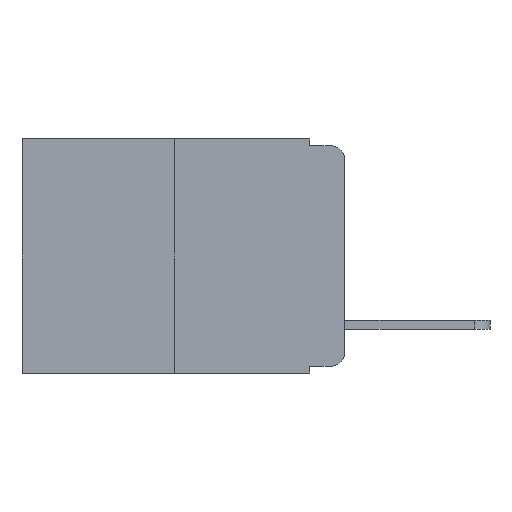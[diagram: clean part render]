
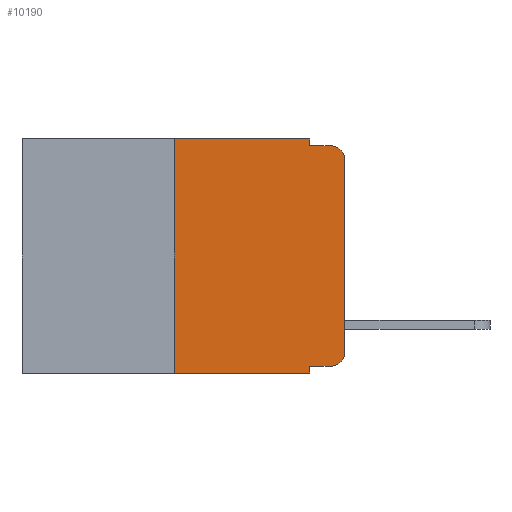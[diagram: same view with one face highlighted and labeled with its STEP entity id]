
A CAD part, left-side view. The second image highlights one B-rep face of the part: STEP entity #10190.
In plain terms, the highlighted planar face has unit normal (-1, 0, 0).
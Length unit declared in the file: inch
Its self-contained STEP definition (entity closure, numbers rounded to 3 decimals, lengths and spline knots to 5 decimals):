
#21 = CARTESIAN_POINT ( 'NONE',  ( 0., 0.051, -0.333 ) ) ;
#350 = LINE ( 'NONE', #20347, #641 ) ;
#398 = VERTEX_POINT ( 'NONE', #1361 ) ;
#641 = VECTOR ( 'NONE', #10774, 39.37008 ) ;
#813 = DIRECTION ( 'NONE',  ( 1., 0., 0. ) ) ;
#1032 = CARTESIAN_POINT ( 'NONE',  ( 0., 0.051, -0.01 ) ) ;
#1087 = DIRECTION ( 'NONE',  ( 0., 0., -1. ) ) ;
#1361 = CARTESIAN_POINT ( 'NONE',  ( 0., 0.02, -0.333 ) ) ;
#1393 = FACE_OUTER_BOUND ( 'NONE', #23180, .T. ) ;
#1511 = LINE ( 'NONE', #2516, #10197 ) ;
#1524 = EDGE_CURVE ( 'NONE', #4655, #13715, #18737, .T. ) ;
#1717 = DIRECTION ( 'NONE',  ( -1., 0., 0. ) ) ;
#1912 = ORIENTED_EDGE ( 'NONE', *, *, #14269, .F. ) ;
#2394 = DIRECTION ( 'NONE',  ( 0., -1., 0. ) ) ;
#2400 = CARTESIAN_POINT ( 'NONE',  ( 0., 0., -0.313 ) ) ;
#2425 = DIRECTION ( 'NONE',  ( 0., 0., -1. ) ) ;
#2516 = CARTESIAN_POINT ( 'NONE',  ( 0., 0.051, 0. ) ) ;
#2588 = DIRECTION ( 'NONE',  ( -1., 0., 0. ) ) ;
#3031 = CARTESIAN_POINT ( 'NONE',  ( 0., 0.25, 0. ) ) ;
#3085 = LINE ( 'NONE', #8792, #3395 ) ;
#3395 = VECTOR ( 'NONE', #6809, 39.37008 ) ;
#3649 = EDGE_CURVE ( 'NONE', #6539, #9116, #3085, .T. ) ;
#4392 = CARTESIAN_POINT ( 'NONE',  ( 0., 0.25, 0. ) ) ;
#4655 = VERTEX_POINT ( 'NONE', #2400 ) ;
#5365 = CARTESIAN_POINT ( 'NONE',  ( 0., 0., -0.03 ) ) ;
#5490 = DIRECTION ( 'NONE',  ( 0., 0., -1. ) ) ;
#6101 = CARTESIAN_POINT ( 'NONE',  ( 0., 0.02, -0.313 ) ) ;
#6539 = VERTEX_POINT ( 'NONE', #22568 ) ;
#6756 = AXIS2_PLACEMENT_3D ( 'NONE', #22762, #1717, #5490 ) ;
#6809 = DIRECTION ( 'NONE',  ( 0., 0., -1. ) ) ;
#6856 = CARTESIAN_POINT ( 'NONE',  ( 0., 0.051, -0.343 ) ) ;
#7246 = LINE ( 'NONE', #3031, #16586 ) ;
#7533 = VECTOR ( 'NONE', #10678, 39.37008 ) ;
#7685 = EDGE_CURVE ( 'NONE', #13715, #15656, #9751, .T. ) ;
#8792 = CARTESIAN_POINT ( 'NONE',  ( 0., 0.051, 0. ) ) ;
#8819 = EDGE_CURVE ( 'NONE', #398, #4655, #23604, .T. ) ;
#8916 = VERTEX_POINT ( 'NONE', #6856 ) ;
#9116 = VERTEX_POINT ( 'NONE', #1032 ) ;
#9135 = CARTESIAN_POINT ( 'NONE',  ( 0., 0.02, -0.01 ) ) ;
#9643 = ORIENTED_EDGE ( 'NONE', *, *, #24073, .F. ) ;
#9751 = CIRCLE ( 'NONE', #6756, 0.02 ) ;
#10037 = DIRECTION ( 'NONE',  ( 0., 0., -1. ) ) ;
#10190 = ADVANCED_FACE ( 'NONE', ( #1393 ), #12395, .F. ) ;
#10197 = VECTOR ( 'NONE', #10037, 39.37008 ) ;
#10291 = CARTESIAN_POINT ( 'NONE',  ( 0., 0.473, 0. ) ) ;
#10678 = DIRECTION ( 'NONE',  ( 0., -1., 0. ) ) ;
#10774 = DIRECTION ( 'NONE',  ( 0., -1., 0. ) ) ;
#11916 = VERTEX_POINT ( 'NONE', #21 ) ;
#12016 = ORIENTED_EDGE ( 'NONE', *, *, #17034, .F. ) ;
#12337 = ORIENTED_EDGE ( 'NONE', *, *, #16049, .T. ) ;
#12395 = PLANE ( 'NONE',  #17717 ) ;
#12532 = DIRECTION ( 'NONE',  ( 0., 0., 1. ) ) ;
#12714 = ORIENTED_EDGE ( 'NONE', *, *, #17772, .T. ) ;
#13476 = LINE ( 'NONE', #13868, #21951 ) ;
#13715 = VERTEX_POINT ( 'NONE', #5365 ) ;
#13868 = CARTESIAN_POINT ( 'NONE',  ( 0., 0.473, 0. ) ) ;
#13963 = AXIS2_PLACEMENT_3D ( 'NONE', #6101, #2588, #2425 ) ;
#14139 = VECTOR ( 'NONE', #12532, 39.37008 ) ;
#14269 = EDGE_CURVE ( 'NONE', #9116, #15656, #18974, .T. ) ;
#14662 = ORIENTED_EDGE ( 'NONE', *, *, #3649, .F. ) ;
#15656 = VERTEX_POINT ( 'NONE', #9135 ) ;
#16022 = ORIENTED_EDGE ( 'NONE', *, *, #8819, .T. ) ;
#16049 = EDGE_CURVE ( 'NONE', #11916, #398, #350, .T. ) ;
#16217 = VECTOR ( 'NONE', #20262, 39.37008 ) ;
#16258 = ORIENTED_EDGE ( 'NONE', *, *, #1524, .T. ) ;
#16586 = VECTOR ( 'NONE', #22487, 39.37008 ) ;
#17034 = EDGE_CURVE ( 'NONE', #11916, #8916, #1511, .T. ) ;
#17676 = VERTEX_POINT ( 'NONE', #4392 ) ;
#17717 = AXIS2_PLACEMENT_3D ( 'NONE', #10291, #813, #1087 ) ;
#17772 = EDGE_CURVE ( 'NONE', #21854, #8916, #21691, .T. ) ;
#18050 = CARTESIAN_POINT ( 'NONE',  ( 0., 0., 0. ) ) ;
#18575 = CARTESIAN_POINT ( 'NONE',  ( 0., 0.473, -0.343 ) ) ;
#18737 = LINE ( 'NONE', #18050, #14139 ) ;
#18974 = LINE ( 'NONE', #22278, #16217 ) ;
#19056 = ORIENTED_EDGE ( 'NONE', *, *, #23083, .F. ) ;
#20262 = DIRECTION ( 'NONE',  ( 0., -1., 0. ) ) ;
#20347 = CARTESIAN_POINT ( 'NONE',  ( 0., 0.051, -0.333 ) ) ;
#20908 = CARTESIAN_POINT ( 'NONE',  ( 0., 0.25, -0.343 ) ) ;
#21691 = LINE ( 'NONE', #18575, #7533 ) ;
#21854 = VERTEX_POINT ( 'NONE', #20908 ) ;
#21951 = VECTOR ( 'NONE', #2394, 39.37008 ) ;
#22278 = CARTESIAN_POINT ( 'NONE',  ( 0., 0.051, -0.01 ) ) ;
#22400 = ORIENTED_EDGE ( 'NONE', *, *, #7685, .T. ) ;
#22487 = DIRECTION ( 'NONE',  ( 0., 0., 1. ) ) ;
#22568 = CARTESIAN_POINT ( 'NONE',  ( 0., 0.051, 0. ) ) ;
#22762 = CARTESIAN_POINT ( 'NONE',  ( 0., 0.02, -0.03 ) ) ;
#23083 = EDGE_CURVE ( 'NONE', #21854, #17676, #7246, .T. ) ;
#23180 = EDGE_LOOP ( 'NONE', ( #16258, #22400, #1912, #14662, #9643, #19056, #12714, #12016, #12337, #16022 ) ) ;
#23604 = CIRCLE ( 'NONE', #13963, 0.02 ) ;
#24073 = EDGE_CURVE ( 'NONE', #17676, #6539, #13476, .T. ) ;
